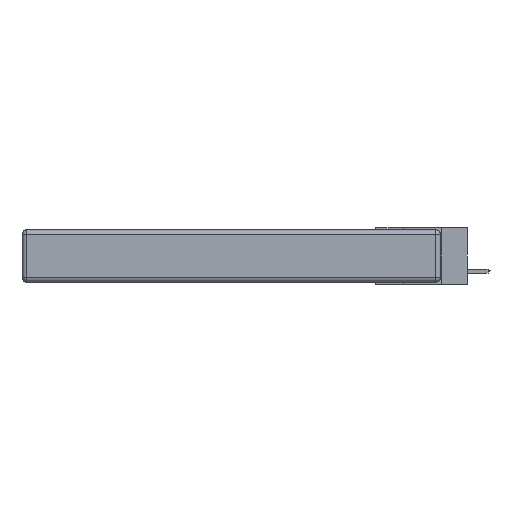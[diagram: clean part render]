
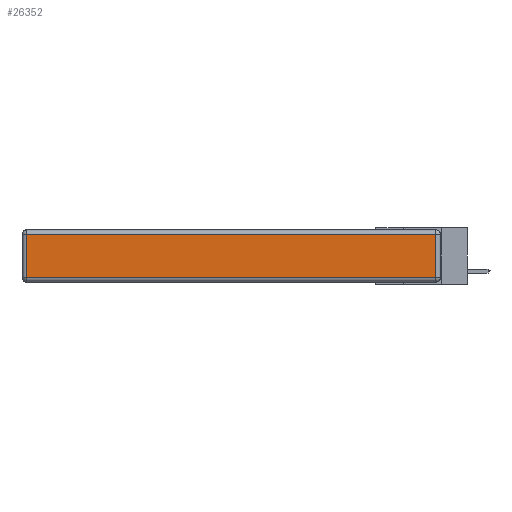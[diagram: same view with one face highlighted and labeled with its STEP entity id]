
A CAD part, left-side view. The second image highlights one B-rep face of the part: STEP entity #26352.
In plain terms, the highlighted planar face has unit normal (-1, 0, 0).
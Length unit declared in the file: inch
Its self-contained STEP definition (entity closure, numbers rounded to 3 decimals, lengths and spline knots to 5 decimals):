
#803 = DIRECTION ( 'NONE',  ( 0., 0., -1. ) ) ;
#955 = PLANE ( 'NONE',  #1667 ) ;
#1158 = ORIENTED_EDGE ( 'NONE', *, *, #5546, .T. ) ;
#1548 = VERTEX_POINT ( 'NONE', #4134 ) ;
#1635 = EDGE_CURVE ( 'NONE', #1548, #10254, #20505, .T. ) ;
#1667 = AXIS2_PLACEMENT_3D ( 'NONE', #4829, #8883, #19293 ) ;
#2842 = EDGE_LOOP ( 'NONE', ( #15223, #1158, #14165, #19086 ) ) ;
#4034 = DIRECTION ( 'NONE',  ( 0., 0., 1. ) ) ;
#4134 = CARTESIAN_POINT ( 'NONE',  ( 0., 2.72, -0.03 ) ) ;
#4697 = FACE_OUTER_BOUND ( 'NONE', #2842, .T. ) ;
#4829 = CARTESIAN_POINT ( 'NONE',  ( 0., 0., -0.343 ) ) ;
#4845 = CARTESIAN_POINT ( 'NONE',  ( 0., 2.72, -0.343 ) ) ;
#5546 = EDGE_CURVE ( 'NONE', #24331, #25205, #21106, .T. ) ;
#5791 = DIRECTION ( 'NONE',  ( 0., 1., 0. ) ) ;
#6593 = VECTOR ( 'NONE', #4034, 39.37008 ) ;
#6817 = CARTESIAN_POINT ( 'NONE',  ( 0., 2.72, -0.313 ) ) ;
#7871 = CARTESIAN_POINT ( 'NONE',  ( 0., 0.03, -0.313 ) ) ;
#8883 = DIRECTION ( 'NONE',  ( -1., 0., 0. ) ) ;
#10254 = VERTEX_POINT ( 'NONE', #6817 ) ;
#14165 = ORIENTED_EDGE ( 'NONE', *, *, #18055, .T. ) ;
#14332 = CARTESIAN_POINT ( 'NONE',  ( 0., 0.03, -0.343 ) ) ;
#15018 = VECTOR ( 'NONE', #803, 39.37008 ) ;
#15223 = ORIENTED_EDGE ( 'NONE', *, *, #17113, .T. ) ;
#16252 = VECTOR ( 'NONE', #5791, 39.37008 ) ;
#17113 = EDGE_CURVE ( 'NONE', #10254, #24331, #18905, .T. ) ;
#18055 = EDGE_CURVE ( 'NONE', #25205, #1548, #20748, .T. ) ;
#18905 = LINE ( 'NONE', #22330, #20503 ) ;
#19086 = ORIENTED_EDGE ( 'NONE', *, *, #1635, .T. ) ;
#19293 = DIRECTION ( 'NONE',  ( 0., 0., 1. ) ) ;
#19564 = CARTESIAN_POINT ( 'NONE',  ( 0., 0.03, -0.03 ) ) ;
#20503 = VECTOR ( 'NONE', #24521, 39.37008 ) ;
#20505 = LINE ( 'NONE', #4845, #15018 ) ;
#20748 = LINE ( 'NONE', #24330, #16252 ) ;
#21106 = LINE ( 'NONE', #14332, #6593 ) ;
#22330 = CARTESIAN_POINT ( 'NONE',  ( 0., 0., -0.313 ) ) ;
#24330 = CARTESIAN_POINT ( 'NONE',  ( 0., 2.75, -0.03 ) ) ;
#24331 = VERTEX_POINT ( 'NONE', #7871 ) ;
#24521 = DIRECTION ( 'NONE',  ( 0., -1., 0. ) ) ;
#25205 = VERTEX_POINT ( 'NONE', #19564 ) ;
#26352 = ADVANCED_FACE ( 'NONE', ( #4697 ), #955, .T. ) ;
